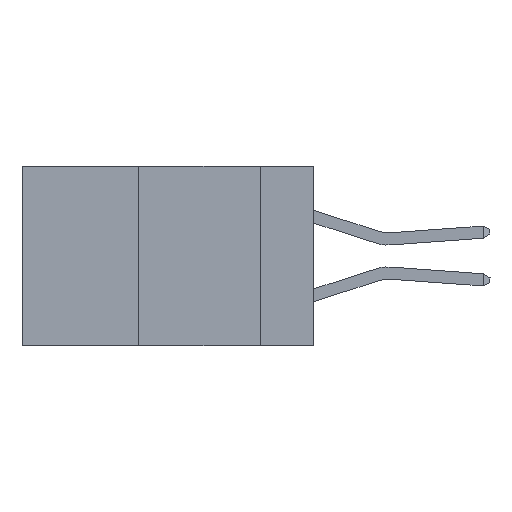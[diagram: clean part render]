
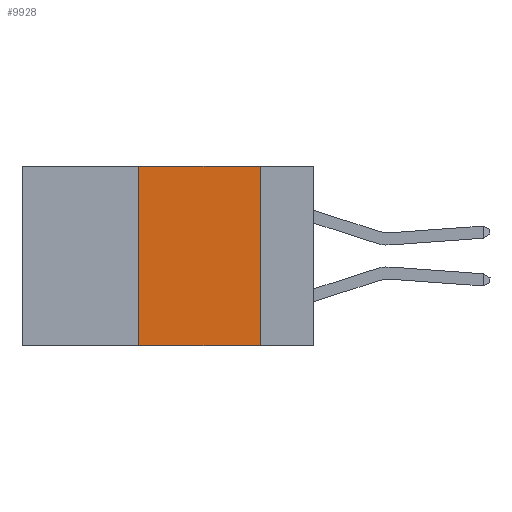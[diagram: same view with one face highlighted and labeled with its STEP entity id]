
A CAD part, left-side view. The second image highlights one B-rep face of the part: STEP entity #9928.
In plain terms, the highlighted planar face has unit normal (-1, 0, 0).
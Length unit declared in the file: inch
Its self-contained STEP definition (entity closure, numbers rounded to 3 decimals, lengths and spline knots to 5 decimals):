
#1090 = CARTESIAN_POINT ( 'NONE',  ( 0., 0.6, 0. ) ) ;
#1520 = EDGE_CURVE ( 'NONE', #22951, #9234, #23018, .T. ) ;
#1566 = DIRECTION ( 'NONE',  ( 1., 0., 0. ) ) ;
#2451 = ORIENTED_EDGE ( 'NONE', *, *, #11817, .F. ) ;
#2540 = DIRECTION ( 'NONE',  ( 0., 0., -1. ) ) ;
#3186 = LINE ( 'NONE', #4534, #9508 ) ;
#4035 = CARTESIAN_POINT ( 'NONE',  ( 0., 0.36, 0. ) ) ;
#4534 = CARTESIAN_POINT ( 'NONE',  ( 0., 0.6, 0. ) ) ;
#6337 = EDGE_LOOP ( 'NONE', ( #21291, #2451, #15753, #21374 ) ) ;
#6654 = LINE ( 'NONE', #17160, #7841 ) ;
#6777 = PLANE ( 'NONE',  #14301 ) ;
#7841 = VECTOR ( 'NONE', #2540, 39.37008 ) ;
#9234 = VERTEX_POINT ( 'NONE', #4035 ) ;
#9508 = VECTOR ( 'NONE', #11924, 39.37008 ) ;
#9866 = CARTESIAN_POINT ( 'NONE',  ( 0., 0.36, 0. ) ) ;
#9928 = ADVANCED_FACE ( 'NONE', ( #14027 ), #6777, .F. ) ;
#11798 = DIRECTION ( 'NONE',  ( 0., 0., 1. ) ) ;
#11817 = EDGE_CURVE ( 'NONE', #9234, #23803, #3186, .T. ) ;
#11924 = DIRECTION ( 'NONE',  ( 0., -1., 0. ) ) ;
#12696 = EDGE_CURVE ( 'NONE', #22951, #21793, #22982, .T. ) ;
#13464 = VECTOR ( 'NONE', #11798, 39.37008 ) ;
#14027 = FACE_OUTER_BOUND ( 'NONE', #6337, .T. ) ;
#14301 = AXIS2_PLACEMENT_3D ( 'NONE', #1090, #1566, #14383 ) ;
#14383 = DIRECTION ( 'NONE',  ( 0., 0., -1. ) ) ;
#15753 = ORIENTED_EDGE ( 'NONE', *, *, #1520, .F. ) ;
#17160 = CARTESIAN_POINT ( 'NONE',  ( 0., 0.11, 0. ) ) ;
#17739 = DIRECTION ( 'NONE',  ( 0., -1., 0. ) ) ;
#19160 = VECTOR ( 'NONE', #17739, 39.37008 ) ;
#19448 = CARTESIAN_POINT ( 'NONE',  ( 0., 0.36, -0.37 ) ) ;
#20984 = CARTESIAN_POINT ( 'NONE',  ( 0., 0.11, 0. ) ) ;
#21291 = ORIENTED_EDGE ( 'NONE', *, *, #21660, .F. ) ;
#21374 = ORIENTED_EDGE ( 'NONE', *, *, #12696, .T. ) ;
#21660 = EDGE_CURVE ( 'NONE', #23803, #21793, #6654, .T. ) ;
#21793 = VERTEX_POINT ( 'NONE', #23793 ) ;
#22867 = CARTESIAN_POINT ( 'NONE',  ( 0., 0.6, -0.37 ) ) ;
#22951 = VERTEX_POINT ( 'NONE', #19448 ) ;
#22982 = LINE ( 'NONE', #22867, #19160 ) ;
#23018 = LINE ( 'NONE', #9866, #13464 ) ;
#23793 = CARTESIAN_POINT ( 'NONE',  ( 0., 0.11, -0.37 ) ) ;
#23803 = VERTEX_POINT ( 'NONE', #20984 ) ;
